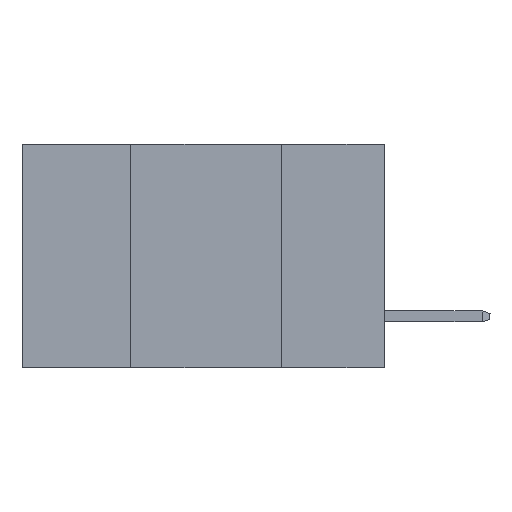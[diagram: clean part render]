
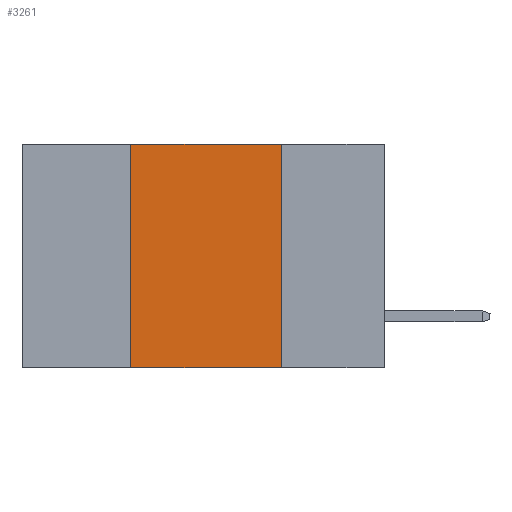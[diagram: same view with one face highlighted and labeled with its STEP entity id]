
A CAD part, left-side view. The second image highlights one B-rep face of the part: STEP entity #3261.
In plain terms, the highlighted planar face has unit normal (-1, 0, 0).
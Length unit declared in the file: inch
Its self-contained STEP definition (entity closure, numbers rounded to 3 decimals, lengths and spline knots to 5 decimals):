
#294 = CARTESIAN_POINT ( 'NONE',  ( 0., 0.6, 0. ) ) ;
#625 = EDGE_CURVE ( 'NONE', #2039, #1903, #6919, .T. ) ;
#635 = VERTEX_POINT ( 'NONE', #5501 ) ;
#809 = EDGE_CURVE ( 'NONE', #635, #7569, #3268, .T. ) ;
#1202 = LINE ( 'NONE', #5827, #4630 ) ;
#1637 = VECTOR ( 'NONE', #5509, 39.37008 ) ;
#1903 = VERTEX_POINT ( 'NONE', #13245 ) ;
#2039 = VERTEX_POINT ( 'NONE', #2138 ) ;
#2138 = CARTESIAN_POINT ( 'NONE',  ( 0., 0.42, -0.37 ) ) ;
#2213 = CARTESIAN_POINT ( 'NONE',  ( 0., 0.6, 0. ) ) ;
#2441 = ORIENTED_EDGE ( 'NONE', *, *, #625, .T. ) ;
#3192 = DIRECTION ( 'NONE',  ( 0., 0., -1. ) ) ;
#3197 = CARTESIAN_POINT ( 'NONE',  ( 0., 0.6, -0.37 ) ) ;
#3261 = ADVANCED_FACE ( 'NONE', ( #3979 ), #7422, .F. ) ;
#3268 = LINE ( 'NONE', #2213, #1637 ) ;
#3979 = FACE_OUTER_BOUND ( 'NONE', #7517, .T. ) ;
#4346 = EDGE_CURVE ( 'NONE', #2039, #635, #1202, .T. ) ;
#4630 = VECTOR ( 'NONE', #4732, 39.37008 ) ;
#4732 = DIRECTION ( 'NONE',  ( 0., 0., 1. ) ) ;
#4875 = DIRECTION ( 'NONE',  ( 1., 0., 0. ) ) ;
#5501 = CARTESIAN_POINT ( 'NONE',  ( 0., 0.42, 0. ) ) ;
#5509 = DIRECTION ( 'NONE',  ( 0., -1., 0. ) ) ;
#5714 = VECTOR ( 'NONE', #3192, 39.37008 ) ;
#5827 = CARTESIAN_POINT ( 'NONE',  ( 0., 0.42, -0.37 ) ) ;
#6765 = CARTESIAN_POINT ( 'NONE',  ( 0., 0.17, -0.37 ) ) ;
#6919 = LINE ( 'NONE', #3197, #9524 ) ;
#7422 = PLANE ( 'NONE',  #7676 ) ;
#7517 = EDGE_LOOP ( 'NONE', ( #10580, #11592, #10857, #2441 ) ) ;
#7569 = VERTEX_POINT ( 'NONE', #13207 ) ;
#7676 = AXIS2_PLACEMENT_3D ( 'NONE', #294, #4875, #14674 ) ;
#9524 = VECTOR ( 'NONE', #12342, 39.37008 ) ;
#10580 = ORIENTED_EDGE ( 'NONE', *, *, #13004, .F. ) ;
#10857 = ORIENTED_EDGE ( 'NONE', *, *, #4346, .F. ) ;
#11120 = LINE ( 'NONE', #6765, #5714 ) ;
#11592 = ORIENTED_EDGE ( 'NONE', *, *, #809, .F. ) ;
#12342 = DIRECTION ( 'NONE',  ( 0., -1., 0. ) ) ;
#13004 = EDGE_CURVE ( 'NONE', #7569, #1903, #11120, .T. ) ;
#13207 = CARTESIAN_POINT ( 'NONE',  ( 0., 0.17, 0. ) ) ;
#13245 = CARTESIAN_POINT ( 'NONE',  ( 0., 0.17, -0.37 ) ) ;
#14674 = DIRECTION ( 'NONE',  ( 0., 0., -1. ) ) ;
